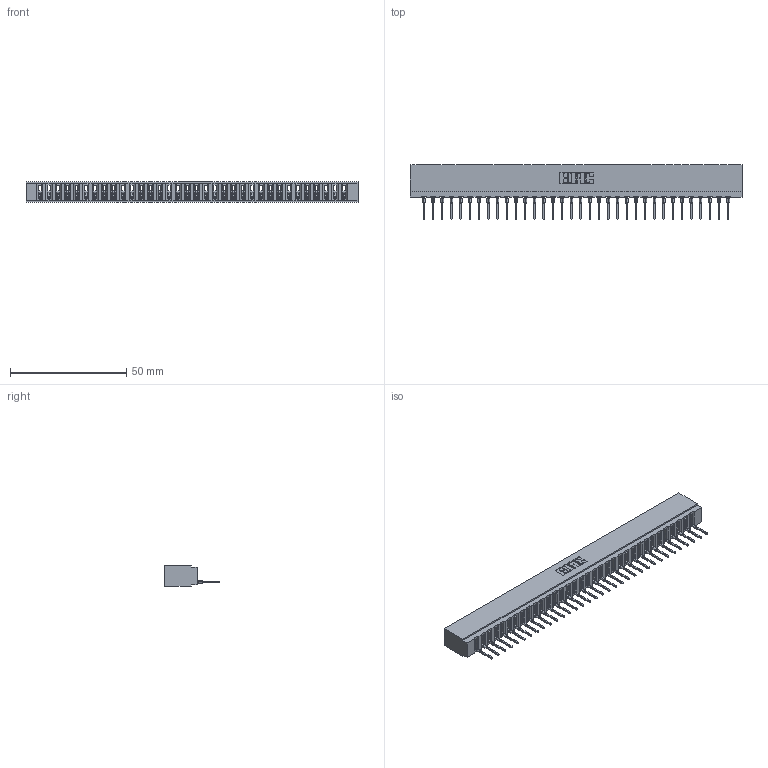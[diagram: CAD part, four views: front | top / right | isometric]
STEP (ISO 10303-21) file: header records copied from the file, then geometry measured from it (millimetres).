
FILE_DESCRIPTION (( 'STEP AP203' ), '1' );
FILE_NAME ('717-034-522-101.STEP', '2026-02-20T21:39:57', ( '' ), ( '' ), 'SwSTEP 2.0', 'SolidWorks 2023', '' );
FILE_SCHEMA (( 'CONFIG_CONTROL_DESIGN' ));
Length unit declared in the file: millimetre
Products named in the file (3): 745-292-001_522; 717-034-522-101; 717 Part_Insulator Option - 06
Assembly tree (35 placements, depth 2):
  717-034-522-101
    717 Part_Insulator Option - 06
    745-292-001_522  x34
Bounding box: 142.6 x 23.48 x 8.89 mm (x, y, z)
Volume: 12091.7 mm3; surface area: 16974.6 mm2
Topology: 35 solids, 35 shells, 3936 faces, 10825 edges, 6830 vertices
Faces by surface type: plane 2366, cylinder 686, bspline 680, torus 204
Entity records: 58297 total; most frequent: CARTESIAN_POINT 10779, ORIENTED_EDGE 10232, DIRECTION 8872, EDGE_CURVE 5116, LINE 4730, VECTOR 4730, VERTEX_POINT 3266, AXIS2_PLACEMENT_3D 2071
